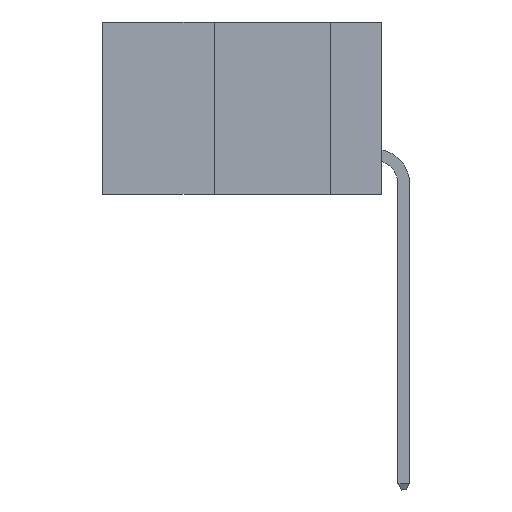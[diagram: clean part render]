
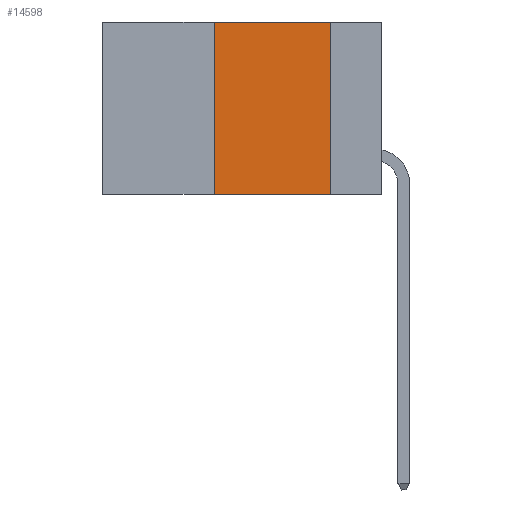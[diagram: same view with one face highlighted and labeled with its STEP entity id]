
A CAD part, left-side view. The second image highlights one B-rep face of the part: STEP entity #14598.
In plain terms, the highlighted planar face has unit normal (-1, 0, 0).
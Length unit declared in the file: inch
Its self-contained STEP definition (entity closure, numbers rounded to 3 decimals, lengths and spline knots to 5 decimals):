
#997 = EDGE_CURVE ( 'NONE', #14256, #19691, #10981, .T. ) ;
#1320 = ORIENTED_EDGE ( 'NONE', *, *, #997, .F. ) ;
#1427 = DIRECTION ( 'NONE',  ( 0., -1., 0. ) ) ;
#2941 = ORIENTED_EDGE ( 'NONE', *, *, #20244, .F. ) ;
#3851 = DIRECTION ( 'NONE',  ( 0., 0., -1. ) ) ;
#5313 = VECTOR ( 'NONE', #1427, 39.37008 ) ;
#5723 = DIRECTION ( 'NONE',  ( 0., 0., -1. ) ) ;
#7037 = DIRECTION ( 'NONE',  ( 0., 0., 1. ) ) ;
#7555 = DIRECTION ( 'NONE',  ( 0., -1., 0. ) ) ;
#7565 = LINE ( 'NONE', #18895, #20453 ) ;
#8163 = CARTESIAN_POINT ( 'NONE',  ( 0., 0.36, 0. ) ) ;
#10981 = LINE ( 'NONE', #17613, #17052 ) ;
#11621 = FACE_OUTER_BOUND ( 'NONE', #12822, .T. ) ;
#12286 = CARTESIAN_POINT ( 'NONE',  ( 0., 0.36, -0.37 ) ) ;
#12822 = EDGE_LOOP ( 'NONE', ( #18164, #1320, #2941, #16325 ) ) ;
#13212 = CARTESIAN_POINT ( 'NONE',  ( 0., 0.6, -0.37 ) ) ;
#13353 = CARTESIAN_POINT ( 'NONE',  ( 0., 0.11, 0. ) ) ;
#14081 = PLANE ( 'NONE',  #15716 ) ;
#14234 = LINE ( 'NONE', #13212, #5313 ) ;
#14256 = VERTEX_POINT ( 'NONE', #8163 ) ;
#14598 = ADVANCED_FACE ( 'NONE', ( #11621 ), #14081, .F. ) ;
#14901 = EDGE_CURVE ( 'NONE', #17073, #19843, #14234, .T. ) ;
#14947 = VECTOR ( 'NONE', #7037, 39.37008 ) ;
#15385 = CARTESIAN_POINT ( 'NONE',  ( 0., 0.36, 0. ) ) ;
#15716 = AXIS2_PLACEMENT_3D ( 'NONE', #20794, #15768, #5723 ) ;
#15768 = DIRECTION ( 'NONE',  ( 1., 0., 0. ) ) ;
#16325 = ORIENTED_EDGE ( 'NONE', *, *, #14901, .T. ) ;
#17032 = EDGE_CURVE ( 'NONE', #19691, #19843, #7565, .T. ) ;
#17052 = VECTOR ( 'NONE', #7555, 39.37008 ) ;
#17073 = VERTEX_POINT ( 'NONE', #12286 ) ;
#17613 = CARTESIAN_POINT ( 'NONE',  ( 0., 0.6, 0. ) ) ;
#17759 = CARTESIAN_POINT ( 'NONE',  ( 0., 0.11, -0.37 ) ) ;
#18164 = ORIENTED_EDGE ( 'NONE', *, *, #17032, .F. ) ;
#18895 = CARTESIAN_POINT ( 'NONE',  ( 0., 0.11, 0. ) ) ;
#19427 = LINE ( 'NONE', #15385, #14947 ) ;
#19691 = VERTEX_POINT ( 'NONE', #13353 ) ;
#19843 = VERTEX_POINT ( 'NONE', #17759 ) ;
#20244 = EDGE_CURVE ( 'NONE', #17073, #14256, #19427, .T. ) ;
#20453 = VECTOR ( 'NONE', #3851, 39.37008 ) ;
#20794 = CARTESIAN_POINT ( 'NONE',  ( 0., 0.6, 0. ) ) ;
